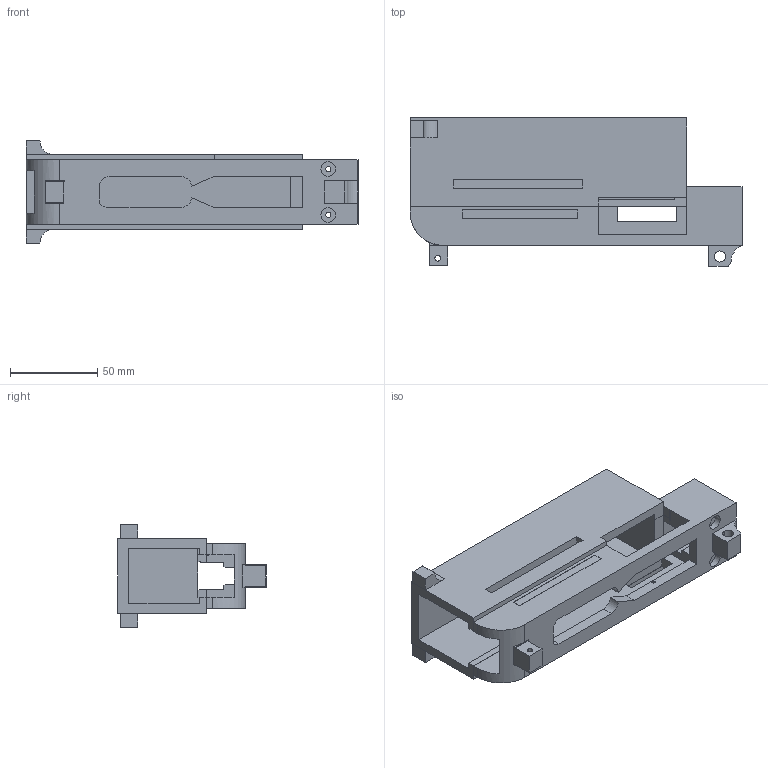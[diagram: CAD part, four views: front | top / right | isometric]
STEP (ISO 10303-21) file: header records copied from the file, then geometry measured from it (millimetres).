
FILE_DESCRIPTION(('FreeCAD Model'),'2;1');
FILE_NAME('shuty v2 upper.step', '2015-07-10T13:27:45',('Author'),(''), 'Open CASCADE STEP processor 6.8','FreeCAD','Unknown');
FILE_SCHEMA(('AUTOMOTIVE_DESIGN_CC2 { 1 2 10303 214 -1 1 5 4 }'));
Length unit declared in the file: millimetre
Products named in the file (1): Pocket017
Bounding box: 190.5 x 84.98 x 59 mm (x, y, z)
Volume: 210221.6 mm3; surface area: 76605.3 mm2
Topology: 1 solids, 1 shells, 151 faces, 458 edges, 309 vertices
Faces by surface type: plane 130, cylinder 21
Full cylindrical faces by diameter (mm): 2 x2, 8 x1, 8.4 x2
Entity records: 11170 total; most frequent: CARTESIAN_POINT 2543, DIRECTION 1422, LINE 1003, VECTOR 1003, ORIENTED_EDGE 916, PCURVE 916, DEFINITIONAL_REPRESENTATION 916, EDGE_CURVE 458
